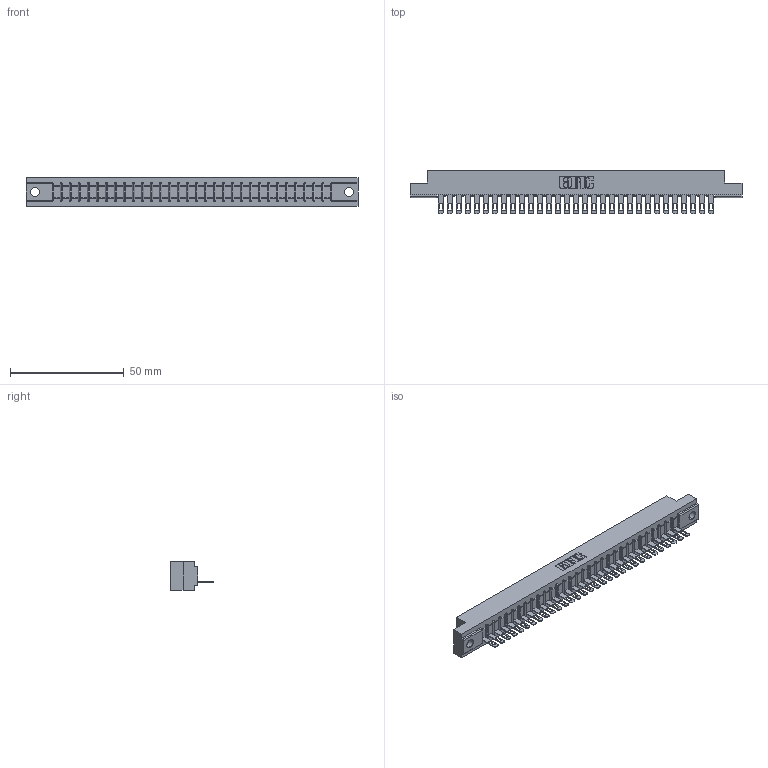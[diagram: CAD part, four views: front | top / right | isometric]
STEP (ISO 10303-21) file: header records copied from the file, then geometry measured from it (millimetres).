
FILE_DESCRIPTION (( 'STEP AP203' ), '1' );
FILE_NAME ('357-031-505-104.STEP', '2018-08-09T22:03:24', ( '' ), ( '' ), 'SwSTEP 2.0', 'SolidWorks 2016', '' );
FILE_SCHEMA (( 'CONFIG_CONTROL_DESIGN' ));
Length unit declared in the file: inch
Products named in the file (3): 307-290-001_505; 357-031-505-104; 307 Part_.156 Dia Mounting Holes
Assembly tree (32 placements, depth 2):
  357-031-505-104
    307 Part_.156 Dia Mounting Holes
    307-290-001_505  x31
Bounding box: 145.85 x 19.18 x 12.7 mm (x, y, z)
Volume: 15014 mm3; surface area: 15849.6 mm2
Topology: 32 solids, 32 shells, 1900 faces, 5381 edges, 3458 vertices
Faces by surface type: plane 1200, cylinder 636, sphere 64
Entity records: 28324 total; most frequent: CARTESIAN_POINT 4770, ORIENTED_EDGE 4754, DIRECTION 4639, EDGE_CURVE 2377, VECTOR 1825, LINE 1825, VERTEX_POINT 1538, AXIS2_PLACEMENT_3D 1407
